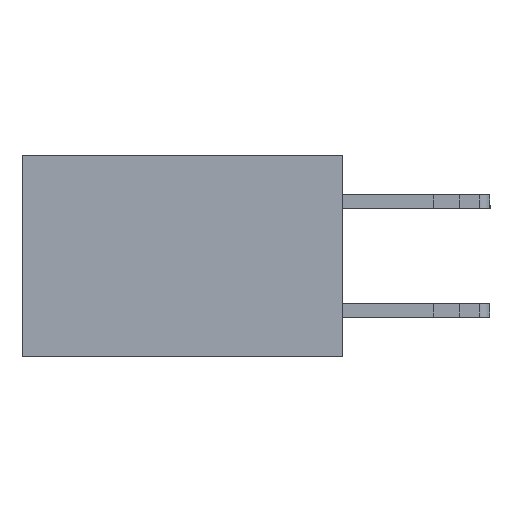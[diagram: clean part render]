
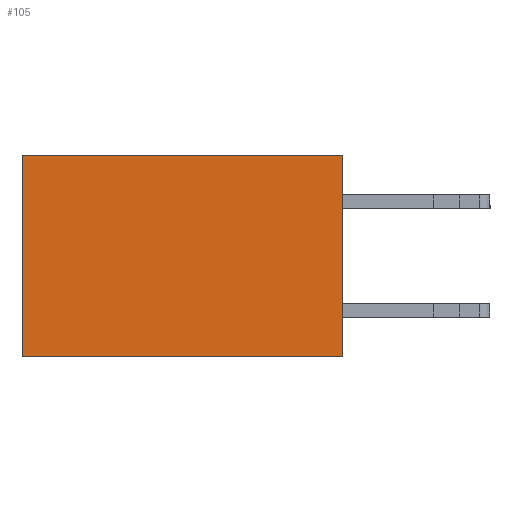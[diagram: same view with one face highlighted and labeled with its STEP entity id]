
A CAD part, left-side view. The second image highlights one B-rep face of the part: STEP entity #105.
In plain terms, the highlighted planar face has unit normal (-1, 0, 0).
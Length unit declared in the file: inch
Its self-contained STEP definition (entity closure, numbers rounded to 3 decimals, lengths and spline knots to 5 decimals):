
#105 = ADVANCED_FACE ( 'NONE', ( #11303 ), #15514, .F. ) ;
#322 = VERTEX_POINT ( 'NONE', #29152 ) ;
#348 = ORIENTED_EDGE ( 'NONE', *, *, #31887, .T. ) ;
#438 = EDGE_LOOP ( 'NONE', ( #15488, #14440, #28907, #348 ) ) ;
#2563 = CARTESIAN_POINT ( 'NONE',  ( 0.277, 0., -0.37 ) ) ;
#3867 = LINE ( 'NONE', #22960, #17199 ) ;
#4669 = EDGE_CURVE ( 'NONE', #25223, #8667, #8359, .T. ) ;
#4877 = CARTESIAN_POINT ( 'NONE',  ( 0.277, 0., -0.37 ) ) ;
#7957 = DIRECTION ( 'NONE',  ( 0., 1., 0. ) ) ;
#8359 = LINE ( 'NONE', #21947, #14250 ) ;
#8425 = CARTESIAN_POINT ( 'NONE',  ( 0.277, 0.59, 0. ) ) ;
#8667 = VERTEX_POINT ( 'NONE', #2563 ) ;
#11303 = FACE_OUTER_BOUND ( 'NONE', #438, .T. ) ;
#12266 = VECTOR ( 'NONE', #30822, 39.37008 ) ;
#13500 = CARTESIAN_POINT ( 'NONE',  ( 0.277, 0.59, -0.37 ) ) ;
#14250 = VECTOR ( 'NONE', #17055, 39.37008 ) ;
#14440 = ORIENTED_EDGE ( 'NONE', *, *, #29122, .F. ) ;
#14681 = LINE ( 'NONE', #4877, #21366 ) ;
#15488 = ORIENTED_EDGE ( 'NONE', *, *, #24945, .T. ) ;
#15505 = CARTESIAN_POINT ( 'NONE',  ( 0.277, 0., -0.37 ) ) ;
#15514 = PLANE ( 'NONE',  #27597 ) ;
#17055 = DIRECTION ( 'NONE',  ( 0., 0., -1. ) ) ;
#17199 = VECTOR ( 'NONE', #7957, 39.37008 ) ;
#21366 = VECTOR ( 'NONE', #22425, 39.37008 ) ;
#21947 = CARTESIAN_POINT ( 'NONE',  ( 0.277, 0., -0.37 ) ) ;
#22425 = DIRECTION ( 'NONE',  ( 0., 1., 0. ) ) ;
#22960 = CARTESIAN_POINT ( 'NONE',  ( 0.277, 0., 0. ) ) ;
#24397 = CARTESIAN_POINT ( 'NONE',  ( 0.277, 0., 0. ) ) ;
#24945 = EDGE_CURVE ( 'NONE', #30688, #322, #31240, .T. ) ;
#25223 = VERTEX_POINT ( 'NONE', #24397 ) ;
#27597 = AXIS2_PLACEMENT_3D ( 'NONE', #15505, #29432, #29322 ) ;
#28907 = ORIENTED_EDGE ( 'NONE', *, *, #4669, .F. ) ;
#29122 = EDGE_CURVE ( 'NONE', #8667, #322, #14681, .T. ) ;
#29152 = CARTESIAN_POINT ( 'NONE',  ( 0.277, 0.59, -0.37 ) ) ;
#29322 = DIRECTION ( 'NONE',  ( 0., 0., -1. ) ) ;
#29432 = DIRECTION ( 'NONE',  ( 1., 0., 0. ) ) ;
#30688 = VERTEX_POINT ( 'NONE', #8425 ) ;
#30822 = DIRECTION ( 'NONE',  ( 0., 0., -1. ) ) ;
#31240 = LINE ( 'NONE', #13500, #12266 ) ;
#31887 = EDGE_CURVE ( 'NONE', #25223, #30688, #3867, .T. ) ;
